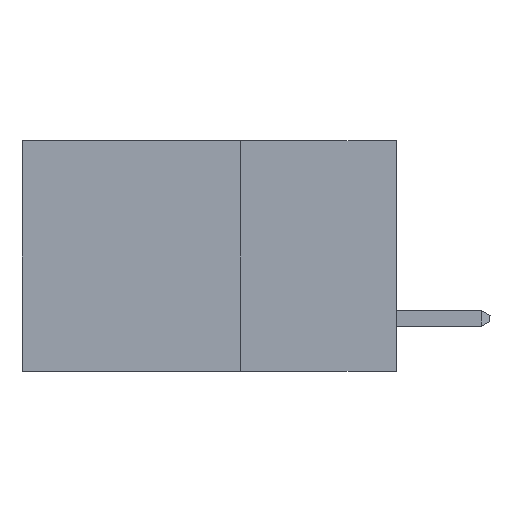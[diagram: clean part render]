
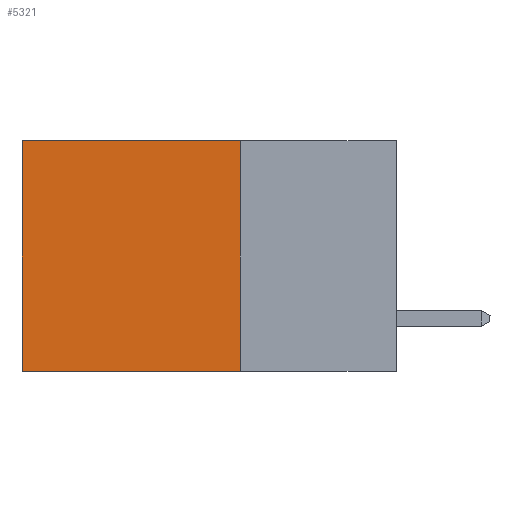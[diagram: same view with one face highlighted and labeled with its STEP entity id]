
A CAD part, left-side view. The second image highlights one B-rep face of the part: STEP entity #5321.
In plain terms, the highlighted planar face has unit normal (-1, 0, 0).
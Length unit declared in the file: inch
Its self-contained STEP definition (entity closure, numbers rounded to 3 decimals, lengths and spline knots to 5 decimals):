
#496 = FACE_OUTER_BOUND ( 'NONE', #7609, .T. ) ;
#1284 = ORIENTED_EDGE ( 'NONE', *, *, #7574, .T. ) ;
#1597 = LINE ( 'NONE', #6337, #7241 ) ;
#1740 = AXIS2_PLACEMENT_3D ( 'NONE', #5341, #8621, #9227 ) ;
#2298 = DIRECTION ( 'NONE',  ( 0., 0., -1. ) ) ;
#2392 = LINE ( 'NONE', #2451, #7422 ) ;
#2451 = CARTESIAN_POINT ( 'NONE',  ( 0.2615, 0.25, -0.37 ) ) ;
#3434 = VECTOR ( 'NONE', #10119, 39.37008 ) ;
#4420 = ORIENTED_EDGE ( 'NONE', *, *, #7063, .T. ) ;
#4799 = ORIENTED_EDGE ( 'NONE', *, *, #5944, .F. ) ;
#4868 = CARTESIAN_POINT ( 'NONE',  ( 0.2615, 0.6, 0. ) ) ;
#4878 = DIRECTION ( 'NONE',  ( 0., 1., 0. ) ) ;
#5026 = VERTEX_POINT ( 'NONE', #4868 ) ;
#5030 = EDGE_CURVE ( 'NONE', #5258, #9976, #1597, .T. ) ;
#5258 = VERTEX_POINT ( 'NONE', #9855 ) ;
#5321 = ADVANCED_FACE ( 'NONE', ( #496 ), #7755, .F. ) ;
#5341 = CARTESIAN_POINT ( 'NONE',  ( 0.2615, 0.25, -0.37 ) ) ;
#5791 = VERTEX_POINT ( 'NONE', #6108 ) ;
#5910 = VECTOR ( 'NONE', #4878, 39.37008 ) ;
#5944 = EDGE_CURVE ( 'NONE', #5791, #5258, #2392, .T. ) ;
#6108 = CARTESIAN_POINT ( 'NONE',  ( 0.2615, 0.25, 0. ) ) ;
#6337 = CARTESIAN_POINT ( 'NONE',  ( 0.2615, 0.25, -0.37 ) ) ;
#6409 = LINE ( 'NONE', #8839, #5910 ) ;
#6854 = LINE ( 'NONE', #8556, #3434 ) ;
#7063 = EDGE_CURVE ( 'NONE', #5026, #9976, #6854, .T. ) ;
#7241 = VECTOR ( 'NONE', #9493, 39.37008 ) ;
#7422 = VECTOR ( 'NONE', #2298, 39.37008 ) ;
#7574 = EDGE_CURVE ( 'NONE', #5791, #5026, #6409, .T. ) ;
#7609 = EDGE_LOOP ( 'NONE', ( #4420, #9859, #4799, #1284 ) ) ;
#7755 = PLANE ( 'NONE',  #1740 ) ;
#7838 = CARTESIAN_POINT ( 'NONE',  ( 0.2615, 0.6, -0.37 ) ) ;
#8556 = CARTESIAN_POINT ( 'NONE',  ( 0.2615, 0.6, -0.37 ) ) ;
#8621 = DIRECTION ( 'NONE',  ( 1., 0., 0. ) ) ;
#8839 = CARTESIAN_POINT ( 'NONE',  ( 0.2615, 0.25, 0. ) ) ;
#9227 = DIRECTION ( 'NONE',  ( 0., 0., -1. ) ) ;
#9493 = DIRECTION ( 'NONE',  ( 0., 1., 0. ) ) ;
#9855 = CARTESIAN_POINT ( 'NONE',  ( 0.2615, 0.25, -0.37 ) ) ;
#9859 = ORIENTED_EDGE ( 'NONE', *, *, #5030, .F. ) ;
#9976 = VERTEX_POINT ( 'NONE', #7838 ) ;
#10119 = DIRECTION ( 'NONE',  ( 0., 0., -1. ) ) ;
